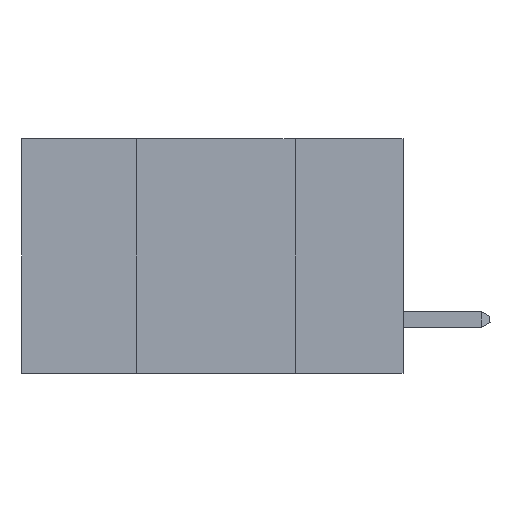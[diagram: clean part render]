
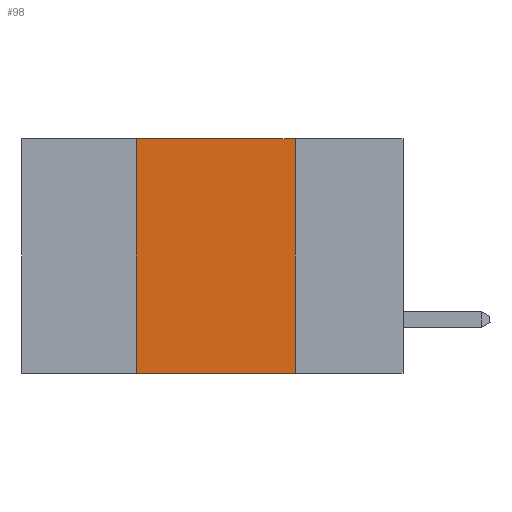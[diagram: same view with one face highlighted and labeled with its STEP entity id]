
A CAD part, left-side view. The second image highlights one B-rep face of the part: STEP entity #98.
In plain terms, the highlighted planar face has unit normal (-1, 0, 0).
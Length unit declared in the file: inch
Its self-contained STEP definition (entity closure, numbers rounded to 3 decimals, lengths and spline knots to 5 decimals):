
#25 = EDGE_CURVE ( 'NONE', #16061, #6975, #11811, .T. ) ;
#98 = ADVANCED_FACE ( 'NONE', ( #18770 ), #12269, .F. ) ;
#712 = EDGE_CURVE ( 'NONE', #6975, #10376, #5829, .T. ) ;
#826 = ORIENTED_EDGE ( 'NONE', *, *, #8741, .T. ) ;
#1956 = ORIENTED_EDGE ( 'NONE', *, *, #25, .F. ) ;
#2354 = DIRECTION ( 'NONE',  ( 0., 0., -1. ) ) ;
#2719 = CARTESIAN_POINT ( 'NONE',  ( 0., 0.42, -0.37 ) ) ;
#2975 = LINE ( 'NONE', #11433, #11683 ) ;
#5051 = DIRECTION ( 'NONE',  ( 0., -1., 0. ) ) ;
#5829 = LINE ( 'NONE', #11515, #13618 ) ;
#5920 = LINE ( 'NONE', #19983, #8018 ) ;
#6975 = VERTEX_POINT ( 'NONE', #11791 ) ;
#8018 = VECTOR ( 'NONE', #16231, 39.37008 ) ;
#8741 = EDGE_CURVE ( 'NONE', #10604, #10376, #2975, .T. ) ;
#8992 = CARTESIAN_POINT ( 'NONE',  ( 0., 0.6, 0. ) ) ;
#10376 = VERTEX_POINT ( 'NONE', #22968 ) ;
#10574 = EDGE_CURVE ( 'NONE', #10604, #16061, #5920, .T. ) ;
#10604 = VERTEX_POINT ( 'NONE', #2719 ) ;
#11096 = DIRECTION ( 'NONE',  ( 0., -1., 0. ) ) ;
#11280 = ORIENTED_EDGE ( 'NONE', *, *, #712, .F. ) ;
#11433 = CARTESIAN_POINT ( 'NONE',  ( 0., 0.6, -0.37 ) ) ;
#11515 = CARTESIAN_POINT ( 'NONE',  ( 0., 0.17, 0. ) ) ;
#11683 = VECTOR ( 'NONE', #11096, 39.37008 ) ;
#11791 = CARTESIAN_POINT ( 'NONE',  ( 0., 0.17, 0. ) ) ;
#11811 = LINE ( 'NONE', #16549, #12741 ) ;
#12269 = PLANE ( 'NONE',  #19475 ) ;
#12611 = DIRECTION ( 'NONE',  ( 0., 0., -1. ) ) ;
#12741 = VECTOR ( 'NONE', #5051, 39.37008 ) ;
#12774 = DIRECTION ( 'NONE',  ( 1., 0., 0. ) ) ;
#13618 = VECTOR ( 'NONE', #2354, 39.37008 ) ;
#15383 = CARTESIAN_POINT ( 'NONE',  ( 0., 0.42, 0. ) ) ;
#16061 = VERTEX_POINT ( 'NONE', #15383 ) ;
#16231 = DIRECTION ( 'NONE',  ( 0., 0., 1. ) ) ;
#16549 = CARTESIAN_POINT ( 'NONE',  ( 0., 0.6, 0. ) ) ;
#18770 = FACE_OUTER_BOUND ( 'NONE', #22053, .T. ) ;
#19475 = AXIS2_PLACEMENT_3D ( 'NONE', #8992, #12774, #12611 ) ;
#19983 = CARTESIAN_POINT ( 'NONE',  ( 0., 0.42, 0. ) ) ;
#22053 = EDGE_LOOP ( 'NONE', ( #11280, #1956, #22279, #826 ) ) ;
#22279 = ORIENTED_EDGE ( 'NONE', *, *, #10574, .F. ) ;
#22968 = CARTESIAN_POINT ( 'NONE',  ( 0., 0.17, -0.37 ) ) ;
